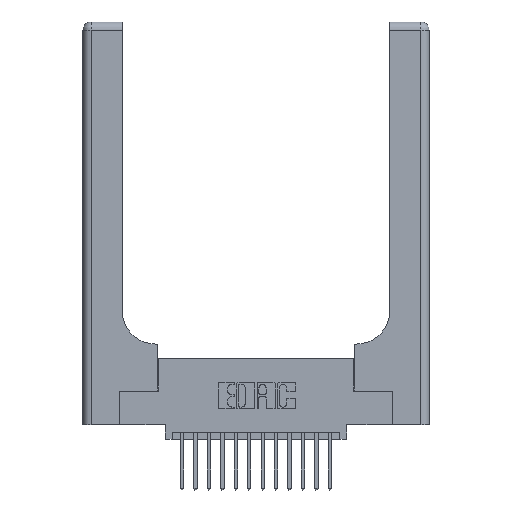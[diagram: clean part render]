
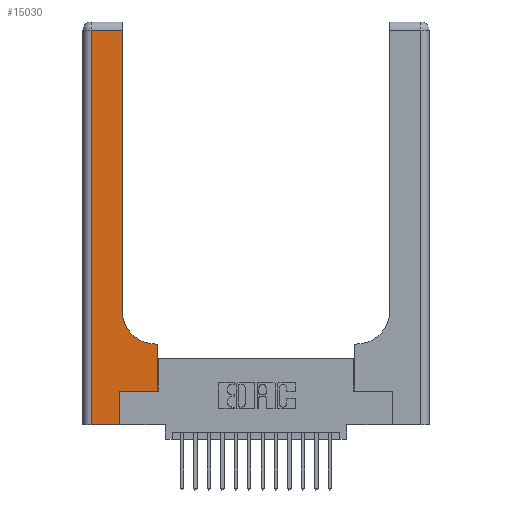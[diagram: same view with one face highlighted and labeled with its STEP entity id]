
A CAD part, top view. The second image highlights one B-rep face of the part: STEP entity #15030.
In plain terms, the highlighted planar face has unit normal (0, 0, 1).
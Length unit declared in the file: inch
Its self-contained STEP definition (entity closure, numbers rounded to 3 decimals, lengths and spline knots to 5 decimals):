
#50 = DIRECTION ( 'NONE',  ( 0., 1., 0. ) ) ;
#571 = CARTESIAN_POINT ( 'NONE',  ( 0.06, 3., 0.37 ) ) ;
#580 = EDGE_CURVE ( 'NONE', #6331, #12857, #15198, .T. ) ;
#885 = CARTESIAN_POINT ( 'NONE',  ( 0., 2.94, 0.37 ) ) ;
#945 = ORIENTED_EDGE ( 'NONE', *, *, #16513, .T. ) ;
#981 = CARTESIAN_POINT ( 'NONE',  ( 0.269, 0., 0.37 ) ) ;
#1272 = VECTOR ( 'NONE', #7466, 39.37008 ) ;
#1694 = EDGE_CURVE ( 'NONE', #2044, #3504, #7325, .T. ) ;
#1787 = AXIS2_PLACEMENT_3D ( 'NONE', #18002, #10934, #2119 ) ;
#1851 = VERTEX_POINT ( 'NONE', #7582 ) ;
#1862 = CIRCLE ( 'NONE', #3081, 0.25 ) ;
#2044 = VERTEX_POINT ( 'NONE', #9975 ) ;
#2057 = PLANE ( 'NONE',  #1787 ) ;
#2067 = ORIENTED_EDGE ( 'NONE', *, *, #6738, .T. ) ;
#2119 = DIRECTION ( 'NONE',  ( -1., 0., 0. ) ) ;
#2931 = VECTOR ( 'NONE', #10725, 39.37008 ) ;
#2964 = EDGE_LOOP ( 'NONE', ( #12057, #10993, #14748, #10791, #2067, #3717, #945, #13712, #7506 ) ) ;
#3081 = AXIS2_PLACEMENT_3D ( 'NONE', #6297, #16350, #7768 ) ;
#3309 = CARTESIAN_POINT ( 'NONE',  ( 0.06, 2.94, 0.37 ) ) ;
#3504 = VERTEX_POINT ( 'NONE', #981 ) ;
#3717 = ORIENTED_EDGE ( 'NONE', *, *, #18119, .T. ) ;
#4201 = EDGE_CURVE ( 'NONE', #12857, #10050, #9751, .T. ) ;
#4236 = CARTESIAN_POINT ( 'NONE',  ( 0.2915, 0.6, 0.37 ) ) ;
#5210 = EDGE_CURVE ( 'NONE', #9329, #6331, #1862, .T. ) ;
#5359 = DIRECTION ( 'NONE',  ( -1., 0., 0. ) ) ;
#5833 = LINE ( 'NONE', #4236, #17305 ) ;
#5858 = VECTOR ( 'NONE', #5359, 39.37008 ) ;
#5915 = CARTESIAN_POINT ( 'NONE',  ( 0.269, 0.25, 0.37 ) ) ;
#6297 = CARTESIAN_POINT ( 'NONE',  ( 0.5415, 0.85, 0.37 ) ) ;
#6331 = VERTEX_POINT ( 'NONE', #18667 ) ;
#6411 = CARTESIAN_POINT ( 'NONE',  ( 0.269, 0.25, 0.37 ) ) ;
#6568 = VECTOR ( 'NONE', #50, 39.37008 ) ;
#6723 = CARTESIAN_POINT ( 'NONE',  ( 0.2915, 3., 0.37 ) ) ;
#6738 = EDGE_CURVE ( 'NONE', #3504, #18373, #12970, .T. ) ;
#6997 = VECTOR ( 'NONE', #15983, 39.37008 ) ;
#7325 = LINE ( 'NONE', #10792, #2931 ) ;
#7466 = DIRECTION ( 'NONE',  ( 0., 1., 0. ) ) ;
#7506 = ORIENTED_EDGE ( 'NONE', *, *, #5210, .T. ) ;
#7582 = CARTESIAN_POINT ( 'NONE',  ( 0.5585, 0.25, 0.37 ) ) ;
#7668 = EDGE_CURVE ( 'NONE', #10050, #2044, #10003, .T. ) ;
#7768 = DIRECTION ( 'NONE',  ( 1., 0., 0. ) ) ;
#8645 = DIRECTION ( 'NONE',  ( -1., 0., 0. ) ) ;
#8741 = DIRECTION ( 'NONE',  ( 0., 1., 0. ) ) ;
#9329 = VERTEX_POINT ( 'NONE', #14335 ) ;
#9380 = EDGE_CURVE ( 'NONE', #11475, #9329, #5833, .T. ) ;
#9751 = LINE ( 'NONE', #885, #5858 ) ;
#9975 = CARTESIAN_POINT ( 'NONE',  ( 0.06, 0., 0.37 ) ) ;
#9991 = LINE ( 'NONE', #17476, #6568 ) ;
#10003 = LINE ( 'NONE', #571, #17133 ) ;
#10050 = VERTEX_POINT ( 'NONE', #3309 ) ;
#10725 = DIRECTION ( 'NONE',  ( 1., 0., 0. ) ) ;
#10791 = ORIENTED_EDGE ( 'NONE', *, *, #1694, .T. ) ;
#10792 = CARTESIAN_POINT ( 'NONE',  ( 0., 0., 0.37 ) ) ;
#10889 = DIRECTION ( 'NONE',  ( 0., -1., 0. ) ) ;
#10934 = DIRECTION ( 'NONE',  ( 0., 0., -1. ) ) ;
#10993 = ORIENTED_EDGE ( 'NONE', *, *, #4201, .T. ) ;
#11435 = VECTOR ( 'NONE', #8741, 39.37008 ) ;
#11475 = VERTEX_POINT ( 'NONE', #14085 ) ;
#12057 = ORIENTED_EDGE ( 'NONE', *, *, #580, .T. ) ;
#12857 = VERTEX_POINT ( 'NONE', #18754 ) ;
#12970 = LINE ( 'NONE', #14626, #1272 ) ;
#13712 = ORIENTED_EDGE ( 'NONE', *, *, #9380, .T. ) ;
#13809 = FACE_OUTER_BOUND ( 'NONE', #2964, .T. ) ;
#14085 = CARTESIAN_POINT ( 'NONE',  ( 0.5585, 0.6, 0.37 ) ) ;
#14335 = CARTESIAN_POINT ( 'NONE',  ( 0.5415, 0.6, 0.37 ) ) ;
#14626 = CARTESIAN_POINT ( 'NONE',  ( 0.269, 0., 0.37 ) ) ;
#14748 = ORIENTED_EDGE ( 'NONE', *, *, #7668, .T. ) ;
#15030 = ADVANCED_FACE ( 'NONE', ( #13809 ), #2057, .F. ) ;
#15198 = LINE ( 'NONE', #6723, #11435 ) ;
#15983 = DIRECTION ( 'NONE',  ( 1., 0., 0. ) ) ;
#16350 = DIRECTION ( 'NONE',  ( 0., 0., -1. ) ) ;
#16513 = EDGE_CURVE ( 'NONE', #1851, #11475, #9991, .T. ) ;
#17133 = VECTOR ( 'NONE', #10889, 39.37008 ) ;
#17305 = VECTOR ( 'NONE', #8645, 39.37008 ) ;
#17476 = CARTESIAN_POINT ( 'NONE',  ( 0.5585, 0.25, 0.37 ) ) ;
#17985 = LINE ( 'NONE', #5915, #6997 ) ;
#18002 = CARTESIAN_POINT ( 'NONE',  ( 0., 3., 0.37 ) ) ;
#18119 = EDGE_CURVE ( 'NONE', #18373, #1851, #17985, .T. ) ;
#18373 = VERTEX_POINT ( 'NONE', #6411 ) ;
#18667 = CARTESIAN_POINT ( 'NONE',  ( 0.2915, 0.85, 0.37 ) ) ;
#18754 = CARTESIAN_POINT ( 'NONE',  ( 0.2915, 2.94, 0.37 ) ) ;
